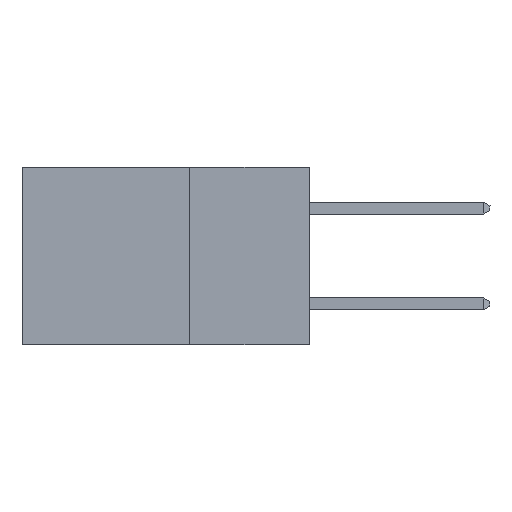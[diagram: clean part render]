
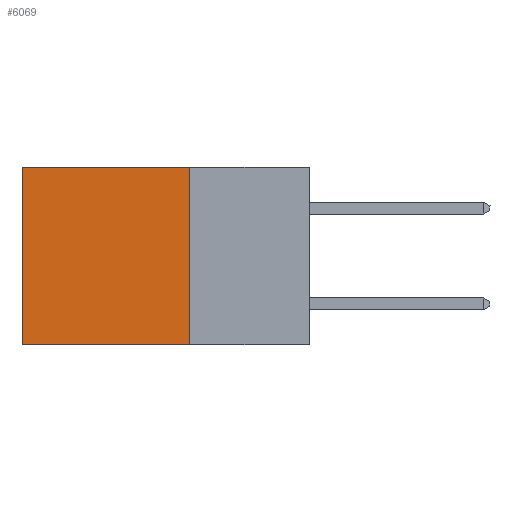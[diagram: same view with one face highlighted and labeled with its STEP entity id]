
A CAD part, left-side view. The second image highlights one B-rep face of the part: STEP entity #6069.
In plain terms, the highlighted planar face has unit normal (-1, 0, 0).
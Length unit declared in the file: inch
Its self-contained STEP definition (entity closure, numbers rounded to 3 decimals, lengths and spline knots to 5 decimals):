
#320 = EDGE_CURVE ( 'NONE', #2967, #12445, #3812, .T. ) ;
#544 = EDGE_CURVE ( 'NONE', #2691, #2967, #6652, .T. ) ;
#568 = DIRECTION ( 'NONE',  ( 0., 1., 0. ) ) ;
#1211 = LINE ( 'NONE', #7094, #8226 ) ;
#1758 = CARTESIAN_POINT ( 'NONE',  ( 0.2875, 0.6, 0. ) ) ;
#2010 = EDGE_CURVE ( 'NONE', #6839, #12445, #3554, .T. ) ;
#2691 = VERTEX_POINT ( 'NONE', #4004 ) ;
#2967 = VERTEX_POINT ( 'NONE', #1758 ) ;
#3554 = LINE ( 'NONE', #5353, #11016 ) ;
#3812 = LINE ( 'NONE', #7961, #11263 ) ;
#4004 = CARTESIAN_POINT ( 'NONE',  ( 0.2875, 0.25, 0. ) ) ;
#4988 = ORIENTED_EDGE ( 'NONE', *, *, #2010, .F. ) ;
#5353 = CARTESIAN_POINT ( 'NONE',  ( 0.2875, 0.25, -0.37 ) ) ;
#5497 = DIRECTION ( 'NONE',  ( 0., 1., 0. ) ) ;
#5752 = DIRECTION ( 'NONE',  ( 0., 0., -1. ) ) ;
#5823 = ORIENTED_EDGE ( 'NONE', *, *, #320, .T. ) ;
#5857 = CARTESIAN_POINT ( 'NONE',  ( 0.2875, 0.25, 0. ) ) ;
#6069 = ADVANCED_FACE ( 'NONE', ( #12516 ), #8632, .F. ) ;
#6652 = LINE ( 'NONE', #5857, #11395 ) ;
#6839 = VERTEX_POINT ( 'NONE', #9710 ) ;
#7094 = CARTESIAN_POINT ( 'NONE',  ( 0.2875, 0.25, 0. ) ) ;
#7376 = ORIENTED_EDGE ( 'NONE', *, *, #8247, .F. ) ;
#7961 = CARTESIAN_POINT ( 'NONE',  ( 0.2875, 0.6, 0. ) ) ;
#8226 = VECTOR ( 'NONE', #11816, 39.37008 ) ;
#8247 = EDGE_CURVE ( 'NONE', #2691, #6839, #1211, .T. ) ;
#8309 = DIRECTION ( 'NONE',  ( 0., 0., -1. ) ) ;
#8632 = PLANE ( 'NONE',  #11287 ) ;
#9192 = CARTESIAN_POINT ( 'NONE',  ( 0.2875, 0.6, -0.37 ) ) ;
#9710 = CARTESIAN_POINT ( 'NONE',  ( 0.2875, 0.25, -0.37 ) ) ;
#11016 = VECTOR ( 'NONE', #568, 39.37008 ) ;
#11263 = VECTOR ( 'NONE', #8309, 39.37008 ) ;
#11287 = AXIS2_PLACEMENT_3D ( 'NONE', #12376, #11473, #5752 ) ;
#11306 = ORIENTED_EDGE ( 'NONE', *, *, #544, .T. ) ;
#11395 = VECTOR ( 'NONE', #5497, 39.37008 ) ;
#11473 = DIRECTION ( 'NONE',  ( 1., 0., 0. ) ) ;
#11816 = DIRECTION ( 'NONE',  ( 0., 0., -1. ) ) ;
#12376 = CARTESIAN_POINT ( 'NONE',  ( 0.2875, 0.25, 0. ) ) ;
#12445 = VERTEX_POINT ( 'NONE', #9192 ) ;
#12516 = FACE_OUTER_BOUND ( 'NONE', #12646, .T. ) ;
#12646 = EDGE_LOOP ( 'NONE', ( #5823, #4988, #7376, #11306 ) ) ;
